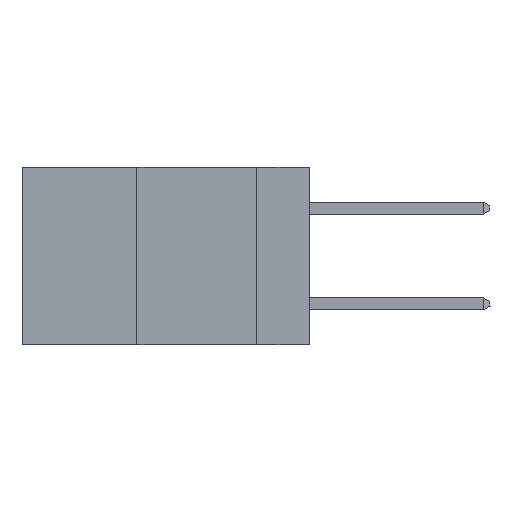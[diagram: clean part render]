
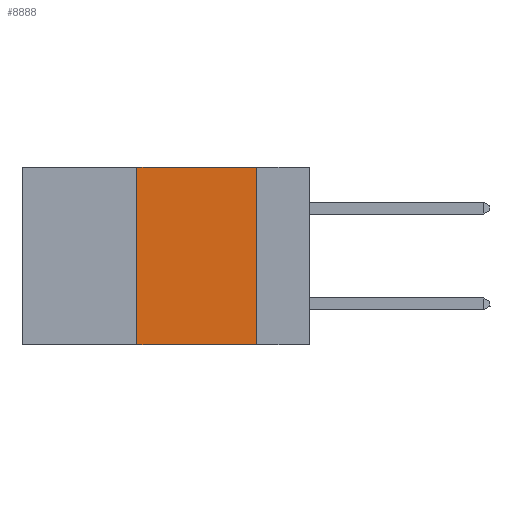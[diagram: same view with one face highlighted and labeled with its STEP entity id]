
A CAD part, left-side view. The second image highlights one B-rep face of the part: STEP entity #8888.
In plain terms, the highlighted planar face has unit normal (-1, 0, 0).
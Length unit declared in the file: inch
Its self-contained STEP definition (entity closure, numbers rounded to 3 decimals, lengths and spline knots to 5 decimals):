
#272 = VERTEX_POINT ( 'NONE', #18740 ) ;
#347 = VECTOR ( 'NONE', #11824, 39.37008 ) ;
#1133 = ORIENTED_EDGE ( 'NONE', *, *, #4725, .F. ) ;
#2640 = VECTOR ( 'NONE', #14214, 39.37008 ) ;
#2723 = ORIENTED_EDGE ( 'NONE', *, *, #8915, .F. ) ;
#3133 = CARTESIAN_POINT ( 'NONE',  ( 0., 0.11, -0.37 ) ) ;
#3256 = EDGE_LOOP ( 'NONE', ( #1133, #2723, #11313, #8581 ) ) ;
#3879 = DIRECTION ( 'NONE',  ( 0., 0., -1. ) ) ;
#4725 = EDGE_CURVE ( 'NONE', #17131, #17531, #11731, .T. ) ;
#5532 = CARTESIAN_POINT ( 'NONE',  ( 0., 0.6, -0.37 ) ) ;
#6167 = EDGE_CURVE ( 'NONE', #11935, #272, #11462, .T. ) ;
#7215 = DIRECTION ( 'NONE',  ( 0., 0., 1. ) ) ;
#7374 = DIRECTION ( 'NONE',  ( 1., 0., 0. ) ) ;
#7472 = PLANE ( 'NONE',  #12906 ) ;
#7961 = LINE ( 'NONE', #10813, #2640 ) ;
#8581 = ORIENTED_EDGE ( 'NONE', *, *, #16506, .T. ) ;
#8888 = ADVANCED_FACE ( 'NONE', ( #17685 ), #7472, .F. ) ;
#8915 = EDGE_CURVE ( 'NONE', #272, #17131, #7961, .T. ) ;
#10472 = LINE ( 'NONE', #5532, #15929 ) ;
#10515 = CARTESIAN_POINT ( 'NONE',  ( 0., 0.11, 0. ) ) ;
#10813 = CARTESIAN_POINT ( 'NONE',  ( 0., 0.6, 0. ) ) ;
#11313 = ORIENTED_EDGE ( 'NONE', *, *, #6167, .F. ) ;
#11462 = LINE ( 'NONE', #13065, #13484 ) ;
#11731 = LINE ( 'NONE', #10515, #347 ) ;
#11824 = DIRECTION ( 'NONE',  ( 0., 0., -1. ) ) ;
#11935 = VERTEX_POINT ( 'NONE', #13525 ) ;
#11974 = DIRECTION ( 'NONE',  ( 0., -1., 0. ) ) ;
#12512 = CARTESIAN_POINT ( 'NONE',  ( 0., 0.11, 0. ) ) ;
#12906 = AXIS2_PLACEMENT_3D ( 'NONE', #13624, #7374, #3879 ) ;
#13065 = CARTESIAN_POINT ( 'NONE',  ( 0., 0.36, 0. ) ) ;
#13484 = VECTOR ( 'NONE', #7215, 39.37008 ) ;
#13525 = CARTESIAN_POINT ( 'NONE',  ( 0., 0.36, -0.37 ) ) ;
#13624 = CARTESIAN_POINT ( 'NONE',  ( 0., 0.6, 0. ) ) ;
#14214 = DIRECTION ( 'NONE',  ( 0., -1., 0. ) ) ;
#15929 = VECTOR ( 'NONE', #11974, 39.37008 ) ;
#16506 = EDGE_CURVE ( 'NONE', #11935, #17531, #10472, .T. ) ;
#17131 = VERTEX_POINT ( 'NONE', #12512 ) ;
#17531 = VERTEX_POINT ( 'NONE', #3133 ) ;
#17685 = FACE_OUTER_BOUND ( 'NONE', #3256, .T. ) ;
#18740 = CARTESIAN_POINT ( 'NONE',  ( 0., 0.36, 0. ) ) ;
